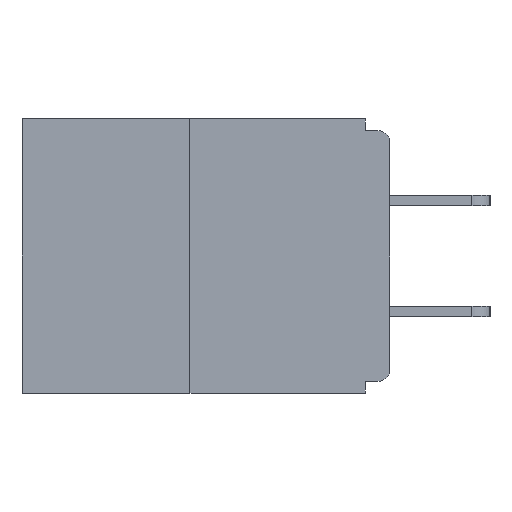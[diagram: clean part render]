
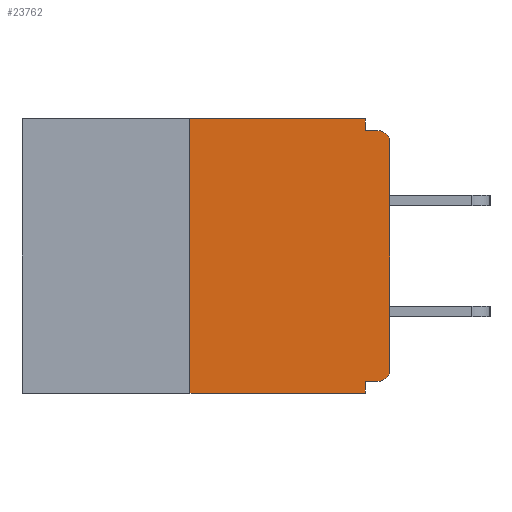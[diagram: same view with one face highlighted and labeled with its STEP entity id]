
A CAD part, left-side view. The second image highlights one B-rep face of the part: STEP entity #23762.
In plain terms, the highlighted planar face has unit normal (-1, 0, 0).
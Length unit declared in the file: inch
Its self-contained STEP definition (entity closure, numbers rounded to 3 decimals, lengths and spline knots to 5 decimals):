
#438 = CARTESIAN_POINT ( 'NONE',  ( 0., 0.46, 0. ) ) ;
#655 = DIRECTION ( 'NONE',  ( 0., 0., -1. ) ) ;
#1899 = VERTEX_POINT ( 'NONE', #21218 ) ;
#1937 = VECTOR ( 'NONE', #8832, 39.37008 ) ;
#2406 = VECTOR ( 'NONE', #20205, 39.37008 ) ;
#2683 = LINE ( 'NONE', #19724, #6131 ) ;
#2805 = EDGE_CURVE ( 'NONE', #5041, #6946, #6571, .T. ) ;
#3146 = CARTESIAN_POINT ( 'NONE',  ( 0., 0., -0.328 ) ) ;
#3277 = VECTOR ( 'NONE', #14919, 39.37008 ) ;
#3832 = CARTESIAN_POINT ( 'NONE',  ( 0., 0.46, 0. ) ) ;
#4189 = EDGE_LOOP ( 'NONE', ( #15913, #22700, #24275, #9211, #14881, #13528, #21764, #22848, #8737, #14104 ) ) ;
#4308 = DIRECTION ( 'NONE',  ( -1., 0., 0. ) ) ;
#4801 = EDGE_CURVE ( 'NONE', #24373, #14915, #5383, .T. ) ;
#5041 = VERTEX_POINT ( 'NONE', #18008 ) ;
#5168 = LINE ( 'NONE', #9310, #11335 ) ;
#5313 = AXIS2_PLACEMENT_3D ( 'NONE', #3832, #13531, #7938 ) ;
#5383 = LINE ( 'NONE', #3146, #18110 ) ;
#5487 = CARTESIAN_POINT ( 'NONE',  ( 0., 0.031, 0. ) ) ;
#5520 = EDGE_CURVE ( 'NONE', #13663, #21754, #14364, .T. ) ;
#5932 = PLANE ( 'NONE',  #5313 ) ;
#6131 = VECTOR ( 'NONE', #655, 39.37008 ) ;
#6259 = EDGE_CURVE ( 'NONE', #21754, #13134, #5168, .T. ) ;
#6571 = LINE ( 'NONE', #8593, #20049 ) ;
#6946 = VERTEX_POINT ( 'NONE', #7757 ) ;
#7567 = EDGE_CURVE ( 'NONE', #5041, #1899, #8983, .T. ) ;
#7640 = CARTESIAN_POINT ( 'NONE',  ( 0., 0.015, -0.313 ) ) ;
#7757 = CARTESIAN_POINT ( 'NONE',  ( 0., 0.031, -0.343 ) ) ;
#7938 = DIRECTION ( 'NONE',  ( 0., 0., -1. ) ) ;
#8593 = CARTESIAN_POINT ( 'NONE',  ( 0., 0.46, -0.343 ) ) ;
#8737 = ORIENTED_EDGE ( 'NONE', *, *, #6259, .F. ) ;
#8832 = DIRECTION ( 'NONE',  ( 0., 0., 1. ) ) ;
#8983 = LINE ( 'NONE', #12835, #1937 ) ;
#9211 = ORIENTED_EDGE ( 'NONE', *, *, #18430, .F. ) ;
#9290 = CARTESIAN_POINT ( 'NONE',  ( 0., 0., -0.313 ) ) ;
#9310 = CARTESIAN_POINT ( 'NONE',  ( 0., 0., -0.015 ) ) ;
#11053 = CARTESIAN_POINT ( 'NONE',  ( 0., 0.031, 0. ) ) ;
#11149 = CARTESIAN_POINT ( 'NONE',  ( 0., 0.031, -0.328 ) ) ;
#11335 = VECTOR ( 'NONE', #20335, 39.37008 ) ;
#12289 = CIRCLE ( 'NONE', #15437, 0.015 ) ;
#12708 = CARTESIAN_POINT ( 'NONE',  ( 0., 0., 0. ) ) ;
#12835 = CARTESIAN_POINT ( 'NONE',  ( 0., 0.25, 0. ) ) ;
#13018 = DIRECTION ( 'NONE',  ( 0., 1., 0. ) ) ;
#13037 = DIRECTION ( 'NONE',  ( -1., 0., 0. ) ) ;
#13134 = VERTEX_POINT ( 'NONE', #14497 ) ;
#13264 = EDGE_CURVE ( 'NONE', #24373, #20641, #12289, .T. ) ;
#13428 = FACE_OUTER_BOUND ( 'NONE', #4189, .T. ) ;
#13528 = ORIENTED_EDGE ( 'NONE', *, *, #13264, .T. ) ;
#13531 = DIRECTION ( 'NONE',  ( 1., 0., 0. ) ) ;
#13663 = VERTEX_POINT ( 'NONE', #5487 ) ;
#13686 = LINE ( 'NONE', #438, #18816 ) ;
#14010 = DIRECTION ( 'NONE',  ( 0., 0., -1. ) ) ;
#14104 = ORIENTED_EDGE ( 'NONE', *, *, #5520, .F. ) ;
#14148 = AXIS2_PLACEMENT_3D ( 'NONE', #21371, #4308, #14010 ) ;
#14364 = LINE ( 'NONE', #11053, #2406 ) ;
#14497 = CARTESIAN_POINT ( 'NONE',  ( 0., 0.015, -0.015 ) ) ;
#14881 = ORIENTED_EDGE ( 'NONE', *, *, #4801, .F. ) ;
#14915 = VERTEX_POINT ( 'NONE', #11149 ) ;
#14919 = DIRECTION ( 'NONE',  ( 0., 0., 1. ) ) ;
#15437 = AXIS2_PLACEMENT_3D ( 'NONE', #7640, #13037, #20571 ) ;
#15913 = ORIENTED_EDGE ( 'NONE', *, *, #23418, .F. ) ;
#16157 = DIRECTION ( 'NONE',  ( 0., -1., 0. ) ) ;
#17319 = CIRCLE ( 'NONE', #14148, 0.015 ) ;
#17784 = CARTESIAN_POINT ( 'NONE',  ( 0., 0.031, -0.015 ) ) ;
#18008 = CARTESIAN_POINT ( 'NONE',  ( 0., 0.25, -0.343 ) ) ;
#18110 = VECTOR ( 'NONE', #13018, 39.37008 ) ;
#18430 = EDGE_CURVE ( 'NONE', #14915, #6946, #2683, .T. ) ;
#18816 = VECTOR ( 'NONE', #21273, 39.37008 ) ;
#19724 = CARTESIAN_POINT ( 'NONE',  ( 0., 0.031, -0.343 ) ) ;
#19914 = EDGE_CURVE ( 'NONE', #23658, #13134, #17319, .T. ) ;
#20049 = VECTOR ( 'NONE', #16157, 39.37008 ) ;
#20205 = DIRECTION ( 'NONE',  ( 0., 0., -1. ) ) ;
#20335 = DIRECTION ( 'NONE',  ( 0., -1., 0. ) ) ;
#20370 = CARTESIAN_POINT ( 'NONE',  ( 0., 0., -0.03 ) ) ;
#20571 = DIRECTION ( 'NONE',  ( 0., 0., -1. ) ) ;
#20641 = VERTEX_POINT ( 'NONE', #9290 ) ;
#21201 = CARTESIAN_POINT ( 'NONE',  ( 0., 0.015, -0.328 ) ) ;
#21218 = CARTESIAN_POINT ( 'NONE',  ( 0., 0.25, 0. ) ) ;
#21273 = DIRECTION ( 'NONE',  ( 0., -1., 0. ) ) ;
#21371 = CARTESIAN_POINT ( 'NONE',  ( 0., 0.015, -0.03 ) ) ;
#21754 = VERTEX_POINT ( 'NONE', #17784 ) ;
#21764 = ORIENTED_EDGE ( 'NONE', *, *, #22436, .T. ) ;
#22436 = EDGE_CURVE ( 'NONE', #20641, #23658, #23882, .T. ) ;
#22700 = ORIENTED_EDGE ( 'NONE', *, *, #7567, .F. ) ;
#22848 = ORIENTED_EDGE ( 'NONE', *, *, #19914, .T. ) ;
#23418 = EDGE_CURVE ( 'NONE', #1899, #13663, #13686, .T. ) ;
#23658 = VERTEX_POINT ( 'NONE', #20370 ) ;
#23762 = ADVANCED_FACE ( 'NONE', ( #13428 ), #5932, .F. ) ;
#23882 = LINE ( 'NONE', #12708, #3277 ) ;
#24275 = ORIENTED_EDGE ( 'NONE', *, *, #2805, .T. ) ;
#24373 = VERTEX_POINT ( 'NONE', #21201 ) ;
